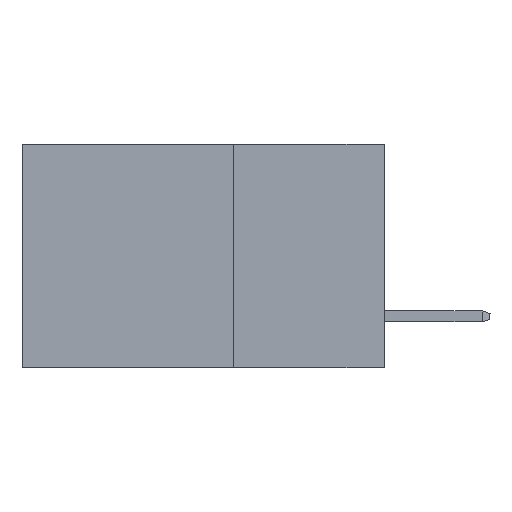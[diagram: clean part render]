
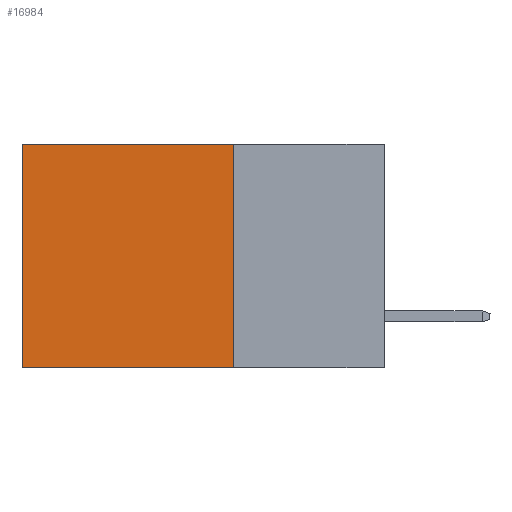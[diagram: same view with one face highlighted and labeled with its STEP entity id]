
A CAD part, left-side view. The second image highlights one B-rep face of the part: STEP entity #16984.
In plain terms, the highlighted planar face has unit normal (-1, 0, 0).
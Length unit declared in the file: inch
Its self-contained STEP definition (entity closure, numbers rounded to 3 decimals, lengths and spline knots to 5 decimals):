
#258 = AXIS2_PLACEMENT_3D ( 'NONE', #14027, #12560, #17610 ) ;
#1366 = VERTEX_POINT ( 'NONE', #9481 ) ;
#1929 = DIRECTION ( 'NONE',  ( 0., 1., 0. ) ) ;
#2008 = EDGE_CURVE ( 'NONE', #4332, #20402, #20412, .T. ) ;
#2193 = EDGE_CURVE ( 'NONE', #1366, #5244, #7534, .T. ) ;
#2424 = VECTOR ( 'NONE', #16374, 39.37008 ) ;
#2735 = VECTOR ( 'NONE', #10705, 39.37008 ) ;
#4332 = VERTEX_POINT ( 'NONE', #5224 ) ;
#4777 = VECTOR ( 'NONE', #1929, 39.37008 ) ;
#5224 = CARTESIAN_POINT ( 'NONE',  ( 0.2615, 0.25, 0. ) ) ;
#5244 = VERTEX_POINT ( 'NONE', #8289 ) ;
#5963 = DIRECTION ( 'NONE',  ( 0., 1., 0. ) ) ;
#6490 = CARTESIAN_POINT ( 'NONE',  ( 0.2615, 0.6, 0. ) ) ;
#6736 = ORIENTED_EDGE ( 'NONE', *, *, #17144, .T. ) ;
#7206 = EDGE_LOOP ( 'NONE', ( #6736, #21308, #19413, #15573 ) ) ;
#7534 = LINE ( 'NONE', #14337, #16931 ) ;
#8289 = CARTESIAN_POINT ( 'NONE',  ( 0.2615, 0.6, -0.37 ) ) ;
#8672 = PLANE ( 'NONE',  #258 ) ;
#9481 = CARTESIAN_POINT ( 'NONE',  ( 0.2615, 0.25, -0.37 ) ) ;
#10705 = DIRECTION ( 'NONE',  ( 0., 0., -1. ) ) ;
#11999 = CARTESIAN_POINT ( 'NONE',  ( 0.2615, 0.25, 0. ) ) ;
#12229 = FACE_OUTER_BOUND ( 'NONE', #7206, .T. ) ;
#12560 = DIRECTION ( 'NONE',  ( 1., 0., 0. ) ) ;
#12662 = CARTESIAN_POINT ( 'NONE',  ( 0.2615, 0.6, -0.37 ) ) ;
#12681 = CARTESIAN_POINT ( 'NONE',  ( 0.2615, 0.25, -0.37 ) ) ;
#12787 = LINE ( 'NONE', #12662, #2424 ) ;
#14027 = CARTESIAN_POINT ( 'NONE',  ( 0.2615, 0.25, -0.37 ) ) ;
#14337 = CARTESIAN_POINT ( 'NONE',  ( 0.2615, 0.25, -0.37 ) ) ;
#15573 = ORIENTED_EDGE ( 'NONE', *, *, #2008, .T. ) ;
#16055 = LINE ( 'NONE', #12681, #2735 ) ;
#16374 = DIRECTION ( 'NONE',  ( 0., 0., -1. ) ) ;
#16931 = VECTOR ( 'NONE', #5963, 39.37008 ) ;
#16984 = ADVANCED_FACE ( 'NONE', ( #12229 ), #8672, .F. ) ;
#17144 = EDGE_CURVE ( 'NONE', #20402, #5244, #12787, .T. ) ;
#17610 = DIRECTION ( 'NONE',  ( 0., 0., -1. ) ) ;
#19413 = ORIENTED_EDGE ( 'NONE', *, *, #19845, .F. ) ;
#19845 = EDGE_CURVE ( 'NONE', #4332, #1366, #16055, .T. ) ;
#20402 = VERTEX_POINT ( 'NONE', #6490 ) ;
#20412 = LINE ( 'NONE', #11999, #4777 ) ;
#21308 = ORIENTED_EDGE ( 'NONE', *, *, #2193, .F. ) ;
